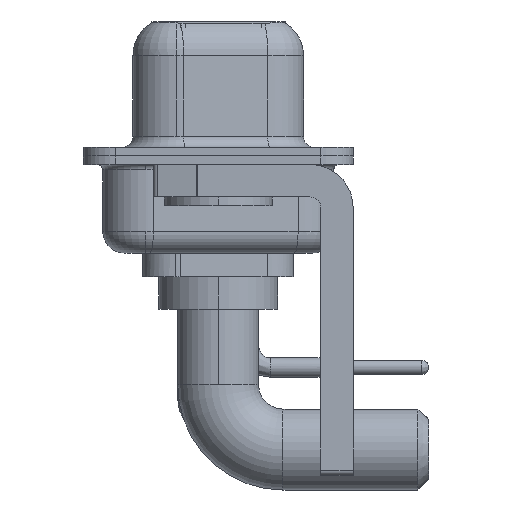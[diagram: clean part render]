
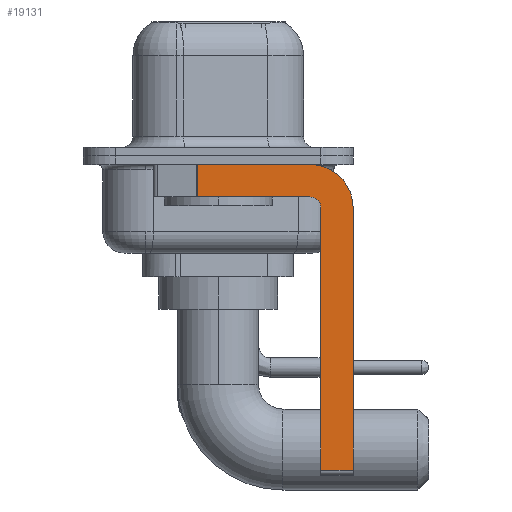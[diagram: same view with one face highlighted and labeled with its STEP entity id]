
A CAD part, left-side view. The second image highlights one B-rep face of the part: STEP entity #19131.
In plain terms, the highlighted planar face has unit normal (-1, 0, 0).
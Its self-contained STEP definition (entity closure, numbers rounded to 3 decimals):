
#116 = FACE_OUTER_BOUND ( 'NONE', #8706, .T. ) ;
#613 = DIRECTION ( 'NONE',  ( 0., -1., 0. ) ) ;
#687 = LINE ( 'NONE', #5336, #3392 ) ;
#1057 = EDGE_CURVE ( 'NONE', #10536, #19210, #18646, .T. ) ;
#1411 = LINE ( 'NONE', #7889, #20025 ) ;
#1920 = VECTOR ( 'NONE', #613, 1000. ) ;
#1922 = EDGE_CURVE ( 'NONE', #18336, #2421, #18986, .T. ) ;
#2421 = VERTEX_POINT ( 'NONE', #18443 ) ;
#2692 = ORIENTED_EDGE ( 'NONE', *, *, #1922, .F. ) ;
#2749 = CARTESIAN_POINT ( 'NONE',  ( -2.9, -4.25, -1.9 ) ) ;
#3195 = ORIENTED_EDGE ( 'NONE', *, *, #1057, .T. ) ;
#3203 = DIRECTION ( 'NONE',  ( 0., 0., -1. ) ) ;
#3392 = VECTOR ( 'NONE', #18309, 1000. ) ;
#3441 = EDGE_CURVE ( 'NONE', #2421, #16478, #9468, .T. ) ;
#3643 = DIRECTION ( 'NONE',  ( 0., 0., 1. ) ) ;
#4226 = ORIENTED_EDGE ( 'NONE', *, *, #15222, .F. ) ;
#4303 = CARTESIAN_POINT ( 'NONE',  ( -2.9, -4.25, -1.9 ) ) ;
#4401 = DIRECTION ( 'NONE',  ( 0., 0., -1. ) ) ;
#4570 = CARTESIAN_POINT ( 'NONE',  ( -2.9, -6.25, -2.4 ) ) ;
#5336 = CARTESIAN_POINT ( 'NONE',  ( -2.9, -4.75, -14.8 ) ) ;
#5514 = ORIENTED_EDGE ( 'NONE', *, *, #14093, .F. ) ;
#6358 = PLANE ( 'NONE',  #20408 ) ;
#6430 = ORIENTED_EDGE ( 'NONE', *, *, #8714, .F. ) ;
#6523 = CARTESIAN_POINT ( 'NONE',  ( -2.9, -4.25, -2.4 ) ) ;
#6631 = CARTESIAN_POINT ( 'NONE',  ( -2.9, -6.25, -2.4 ) ) ;
#6706 = CARTESIAN_POINT ( 'NONE',  ( -2.9, 0.978, -1.9 ) ) ;
#7194 = CARTESIAN_POINT ( 'NONE',  ( -2.9, -6.25, -14.55 ) ) ;
#7242 = CARTESIAN_POINT ( 'NONE',  ( -2.9, 0.978, -0.4 ) ) ;
#7609 = CARTESIAN_POINT ( 'NONE',  ( -2.9, -4.25, -2.4 ) ) ;
#7889 = CARTESIAN_POINT ( 'NONE',  ( -2.9, 0.978, -1.9 ) ) ;
#7959 = VERTEX_POINT ( 'NONE', #16562 ) ;
#8277 = DIRECTION ( 'NONE',  ( 1., 0., 0. ) ) ;
#8640 = AXIS2_PLACEMENT_3D ( 'NONE', #6523, #11619, #3643 ) ;
#8706 = EDGE_LOOP ( 'NONE', ( #2692, #18897, #5514, #6430, #4226, #3195, #15315, #19853 ) ) ;
#8714 = EDGE_CURVE ( 'NONE', #7959, #11788, #10321, .T. ) ;
#9153 = DIRECTION ( 'NONE',  ( 0., 0., -1. ) ) ;
#9468 = CIRCLE ( 'NONE', #17612, 2. ) ;
#9795 = VECTOR ( 'NONE', #12520, 1000. ) ;
#10321 = CIRCLE ( 'NONE', #8640, 0.5 ) ;
#10492 = DIRECTION ( 'NONE',  ( 0., -1., 0. ) ) ;
#10536 = VERTEX_POINT ( 'NONE', #13917 ) ;
#10639 = LINE ( 'NONE', #4570, #13294 ) ;
#11619 = DIRECTION ( 'NONE',  ( -1., 0., 0. ) ) ;
#11788 = VERTEX_POINT ( 'NONE', #4303 ) ;
#12193 = CARTESIAN_POINT ( 'NONE',  ( -2.9, 3., -0.4 ) ) ;
#12520 = DIRECTION ( 'NONE',  ( 0., 1., 0. ) ) ;
#13294 = VECTOR ( 'NONE', #9153, 1000. ) ;
#13917 = CARTESIAN_POINT ( 'NONE',  ( -2.9, -4.75, -14.55 ) ) ;
#14093 = EDGE_CURVE ( 'NONE', #11788, #20020, #17214, .T. ) ;
#15222 = EDGE_CURVE ( 'NONE', #10536, #7959, #687, .T. ) ;
#15315 = ORIENTED_EDGE ( 'NONE', *, *, #18439, .F. ) ;
#15464 = EDGE_CURVE ( 'NONE', #18336, #20020, #1411, .T. ) ;
#16478 = VERTEX_POINT ( 'NONE', #6631 ) ;
#16562 = CARTESIAN_POINT ( 'NONE',  ( -2.9, -4.75, -2.4 ) ) ;
#17214 = LINE ( 'NONE', #2749, #9795 ) ;
#17612 = AXIS2_PLACEMENT_3D ( 'NONE', #7609, #18969, #4401 ) ;
#18040 = CARTESIAN_POINT ( 'NONE',  ( -2.9, -4.25, -2.4 ) ) ;
#18309 = DIRECTION ( 'NONE',  ( 0., 0., 1. ) ) ;
#18336 = VERTEX_POINT ( 'NONE', #7242 ) ;
#18439 = EDGE_CURVE ( 'NONE', #16478, #19210, #10639, .T. ) ;
#18443 = CARTESIAN_POINT ( 'NONE',  ( -2.9, -4.25, -0.4 ) ) ;
#18646 = LINE ( 'NONE', #20132, #1920 ) ;
#18897 = ORIENTED_EDGE ( 'NONE', *, *, #15464, .T. ) ;
#18969 = DIRECTION ( 'NONE',  ( 1., 0., 0. ) ) ;
#18986 = LINE ( 'NONE', #12193, #20231 ) ;
#19131 = ADVANCED_FACE ( 'NONE', ( #116 ), #6358, .F. ) ;
#19210 = VERTEX_POINT ( 'NONE', #7194 ) ;
#19329 = DIRECTION ( 'NONE',  ( 0., 0., -1. ) ) ;
#19853 = ORIENTED_EDGE ( 'NONE', *, *, #3441, .F. ) ;
#20020 = VERTEX_POINT ( 'NONE', #6706 ) ;
#20025 = VECTOR ( 'NONE', #3203, 1000. ) ;
#20132 = CARTESIAN_POINT ( 'NONE',  ( -2.9, -4.25, -14.55 ) ) ;
#20231 = VECTOR ( 'NONE', #10492, 1000. ) ;
#20408 = AXIS2_PLACEMENT_3D ( 'NONE', #18040, #8277, #19329 ) ;
